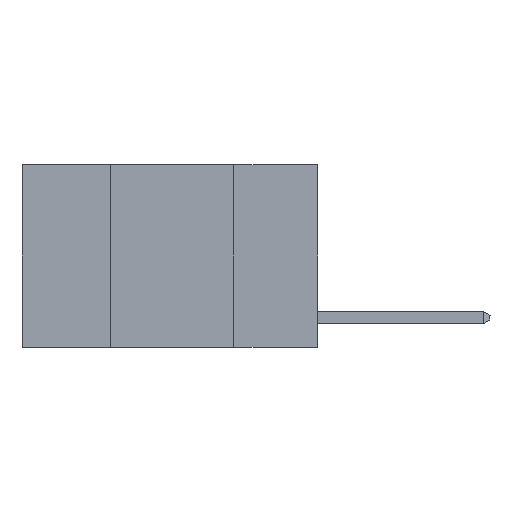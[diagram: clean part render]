
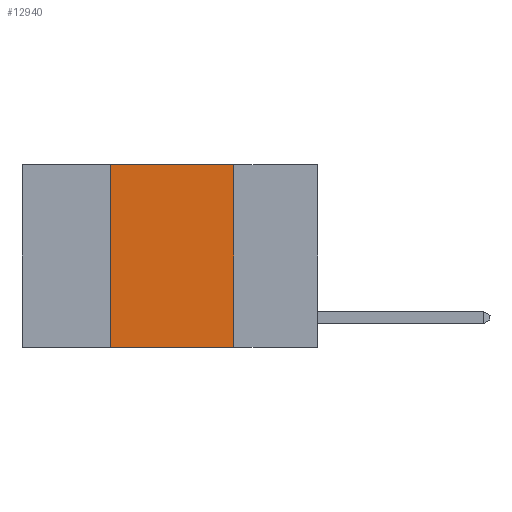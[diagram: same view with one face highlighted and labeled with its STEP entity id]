
A CAD part, left-side view. The second image highlights one B-rep face of the part: STEP entity #12940.
In plain terms, the highlighted planar face has unit normal (-1, 0, 0).
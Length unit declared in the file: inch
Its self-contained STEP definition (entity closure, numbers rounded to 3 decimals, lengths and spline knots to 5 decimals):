
#84 = CARTESIAN_POINT ( 'NONE',  ( 0., 0.42, 0. ) ) ;
#392 = ORIENTED_EDGE ( 'NONE', *, *, #3837, .F. ) ;
#495 = LINE ( 'NONE', #9187, #2411 ) ;
#692 = ORIENTED_EDGE ( 'NONE', *, *, #2664, .F. ) ;
#766 = DIRECTION ( 'NONE',  ( 0., -1., 0. ) ) ;
#807 = PLANE ( 'NONE',  #10046 ) ;
#946 = DIRECTION ( 'NONE',  ( 1., 0., 0. ) ) ;
#1515 = LINE ( 'NONE', #9016, #6583 ) ;
#1679 = VERTEX_POINT ( 'NONE', #7723 ) ;
#2411 = VECTOR ( 'NONE', #766, 39.37008 ) ;
#2664 = EDGE_CURVE ( 'NONE', #4521, #12064, #4706, .T. ) ;
#3021 = LINE ( 'NONE', #13782, #7423 ) ;
#3090 = DIRECTION ( 'NONE',  ( 0., 0., -1. ) ) ;
#3837 = EDGE_CURVE ( 'NONE', #12064, #8390, #3021, .T. ) ;
#4521 = VERTEX_POINT ( 'NONE', #8110 ) ;
#4706 = LINE ( 'NONE', #8058, #11812 ) ;
#6061 = EDGE_CURVE ( 'NONE', #4521, #1679, #495, .T. ) ;
#6583 = VECTOR ( 'NONE', #13439, 39.37008 ) ;
#6910 = EDGE_LOOP ( 'NONE', ( #8818, #392, #692, #12393 ) ) ;
#7423 = VECTOR ( 'NONE', #12713, 39.37008 ) ;
#7723 = CARTESIAN_POINT ( 'NONE',  ( 0., 0.17, -0.37 ) ) ;
#8058 = CARTESIAN_POINT ( 'NONE',  ( 0., 0.42, 0. ) ) ;
#8110 = CARTESIAN_POINT ( 'NONE',  ( 0., 0.42, -0.37 ) ) ;
#8390 = VERTEX_POINT ( 'NONE', #8643 ) ;
#8643 = CARTESIAN_POINT ( 'NONE',  ( 0., 0.17, 0. ) ) ;
#8818 = ORIENTED_EDGE ( 'NONE', *, *, #11446, .F. ) ;
#9016 = CARTESIAN_POINT ( 'NONE',  ( 0., 0.17, 0. ) ) ;
#9187 = CARTESIAN_POINT ( 'NONE',  ( 0., 0.6, -0.37 ) ) ;
#9651 = CARTESIAN_POINT ( 'NONE',  ( 0., 0.6, 0. ) ) ;
#10046 = AXIS2_PLACEMENT_3D ( 'NONE', #9651, #946, #3090 ) ;
#10647 = FACE_OUTER_BOUND ( 'NONE', #6910, .T. ) ;
#11446 = EDGE_CURVE ( 'NONE', #8390, #1679, #1515, .T. ) ;
#11812 = VECTOR ( 'NONE', #12416, 39.37008 ) ;
#12064 = VERTEX_POINT ( 'NONE', #84 ) ;
#12393 = ORIENTED_EDGE ( 'NONE', *, *, #6061, .T. ) ;
#12416 = DIRECTION ( 'NONE',  ( 0., 0., 1. ) ) ;
#12713 = DIRECTION ( 'NONE',  ( 0., -1., 0. ) ) ;
#12940 = ADVANCED_FACE ( 'NONE', ( #10647 ), #807, .F. ) ;
#13439 = DIRECTION ( 'NONE',  ( 0., 0., -1. ) ) ;
#13782 = CARTESIAN_POINT ( 'NONE',  ( 0., 0.6, 0. ) ) ;
